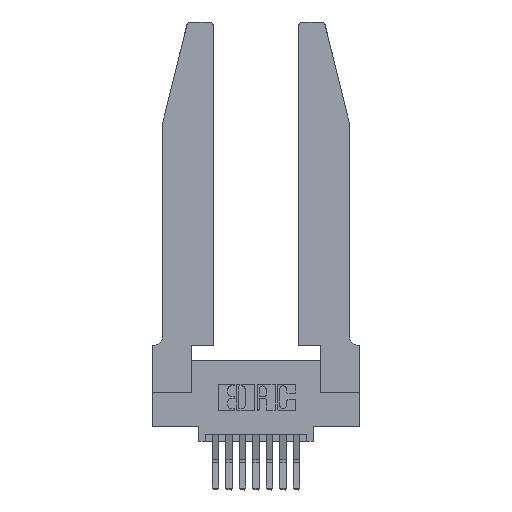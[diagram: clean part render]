
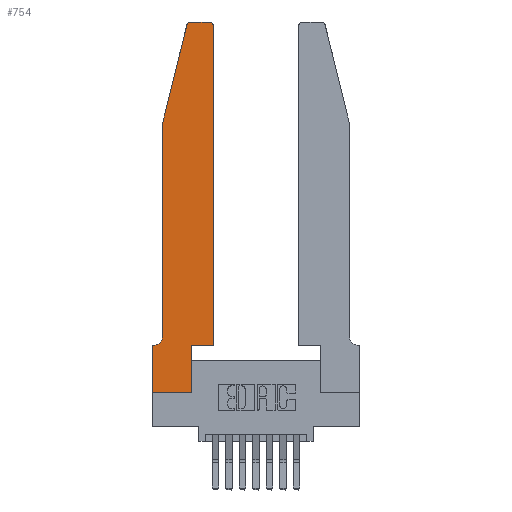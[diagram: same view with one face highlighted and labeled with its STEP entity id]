
A CAD part, top view. The second image highlights one B-rep face of the part: STEP entity #754.
In plain terms, the highlighted planar face has unit normal (0, 0, 1).
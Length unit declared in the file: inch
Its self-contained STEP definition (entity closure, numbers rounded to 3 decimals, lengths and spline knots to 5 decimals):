
#336 = VERTEX_POINT ( 'NONE', #6497 ) ;
#641 = ORIENTED_EDGE ( 'NONE', *, *, #11250, .T. ) ;
#754 = ADVANCED_FACE ( 'NONE', ( #6188 ), #2281, .T. ) ;
#1033 = ORIENTED_EDGE ( 'NONE', *, *, #3215, .T. ) ;
#1109 = EDGE_CURVE ( 'NONE', #2822, #13515, #5227, .T. ) ;
#1657 = CARTESIAN_POINT ( 'NONE',  ( 0.25487, 2.72718, 0.37 ) ) ;
#1688 = CARTESIAN_POINT ( 'NONE',  ( 0.0755, 0.35, 0.37 ) ) ;
#1771 = CARTESIAN_POINT ( 'NONE',  ( 0.4505, 0.35, 0.37 ) ) ;
#2052 = CARTESIAN_POINT ( 'NONE',  ( 0.4505, 2.72, 0.37 ) ) ;
#2219 = DIRECTION ( 'NONE',  ( 0., 0., -1. ) ) ;
#2222 = DIRECTION ( 'NONE',  ( 0., 0., 1. ) ) ;
#2240 = VECTOR ( 'NONE', #10728, 39.37008 ) ;
#2281 = PLANE ( 'NONE',  #11342 ) ;
#2646 = CARTESIAN_POINT ( 'NONE',  ( 0.284, 2.72, 0.37 ) ) ;
#2689 = VERTEX_POINT ( 'NONE', #2052 ) ;
#2822 = VERTEX_POINT ( 'NONE', #8727 ) ;
#2857 = CARTESIAN_POINT ( 'NONE',  ( 0., 0., 0.37 ) ) ;
#2932 = CARTESIAN_POINT ( 'NONE',  ( 0.4505, 0.35, 0.37 ) ) ;
#3115 = VERTEX_POINT ( 'NONE', #13414 ) ;
#3215 = EDGE_CURVE ( 'NONE', #3642, #12084, #13689, .T. ) ;
#3252 = CARTESIAN_POINT ( 'NONE',  ( 0.4205, 2.72, 0.37 ) ) ;
#3642 = VERTEX_POINT ( 'NONE', #1657 ) ;
#3873 = DIRECTION ( 'NONE',  ( 1., 0., 0. ) ) ;
#3960 = CARTESIAN_POINT ( 'NONE',  ( 0.4505, 0.35, 0.37 ) ) ;
#3964 = DIRECTION ( 'NONE',  ( 0., -1., 0. ) ) ;
#4013 = DIRECTION ( 'NONE',  ( 1., 0., 0. ) ) ;
#4084 = CIRCLE ( 'NONE', #13754, 0.03 ) ;
#4226 = ORIENTED_EDGE ( 'NONE', *, *, #5120, .T. ) ;
#4238 = CARTESIAN_POINT ( 'NONE',  ( 0.0055, 0.35, 0.37 ) ) ;
#4379 = LINE ( 'NONE', #8382, #13118 ) ;
#4435 = CARTESIAN_POINT ( 'NONE',  ( 0.2605, 2.75, 0.37 ) ) ;
#4442 = EDGE_CURVE ( 'NONE', #12084, #2822, #4379, .T. ) ;
#4458 = DIRECTION ( 'NONE',  ( 1., 0., 0. ) ) ;
#4613 = VECTOR ( 'NONE', #11310, 39.37008 ) ;
#4625 = VERTEX_POINT ( 'NONE', #10984 ) ;
#5120 = EDGE_CURVE ( 'NONE', #4625, #336, #8622, .T. ) ;
#5227 = CIRCLE ( 'NONE', #13986, 0.07 ) ;
#5838 = EDGE_CURVE ( 'NONE', #336, #7082, #13028, .T. ) ;
#5891 = VERTEX_POINT ( 'NONE', #2857 ) ;
#6188 = FACE_OUTER_BOUND ( 'NONE', #10851, .T. ) ;
#6319 = ORIENTED_EDGE ( 'NONE', *, *, #14062, .T. ) ;
#6497 = CARTESIAN_POINT ( 'NONE',  ( 0.2865, 0.35, 0.37 ) ) ;
#6561 = EDGE_CURVE ( 'NONE', #7082, #2689, #7243, .T. ) ;
#6595 = LINE ( 'NONE', #10935, #12585 ) ;
#6821 = DIRECTION ( 'NONE',  ( -1., 0., 0. ) ) ;
#6855 = CARTESIAN_POINT ( 'NONE',  ( 0.0755, 2., 0.37 ) ) ;
#7029 = EDGE_CURVE ( 'NONE', #7751, #3642, #7226, .T. ) ;
#7069 = CARTESIAN_POINT ( 'NONE',  ( 0.4205, 2.75, 0.37 ) ) ;
#7082 = VERTEX_POINT ( 'NONE', #2932 ) ;
#7086 = VECTOR ( 'NONE', #4013, 39.37008 ) ;
#7226 = CIRCLE ( 'NONE', #8506, 0.03 ) ;
#7243 = LINE ( 'NONE', #1771, #10285 ) ;
#7295 = CARTESIAN_POINT ( 'NONE',  ( 0.2865, 0.35, 0.37 ) ) ;
#7328 = DIRECTION ( 'NONE',  ( 1., 0., 0. ) ) ;
#7700 = LINE ( 'NONE', #1688, #13290 ) ;
#7751 = VERTEX_POINT ( 'NONE', #7919 ) ;
#7878 = CARTESIAN_POINT ( 'NONE',  ( 0.0755, 2., 0.37 ) ) ;
#7919 = CARTESIAN_POINT ( 'NONE',  ( 0.284, 2.75, 0.37 ) ) ;
#8382 = CARTESIAN_POINT ( 'NONE',  ( 0.0755, 2., 0.37 ) ) ;
#8506 = AXIS2_PLACEMENT_3D ( 'NONE', #2646, #10848, #3873 ) ;
#8622 = LINE ( 'NONE', #7295, #2240 ) ;
#8727 = CARTESIAN_POINT ( 'NONE',  ( 0.0755, 0.42, 0.37 ) ) ;
#8882 = VERTEX_POINT ( 'NONE', #7069 ) ;
#9174 = LINE ( 'NONE', #11056, #14657 ) ;
#9280 = EDGE_CURVE ( 'NONE', #5891, #4625, #9174, .T. ) ;
#9311 = VECTOR ( 'NONE', #11351, 39.37008 ) ;
#9752 = ORIENTED_EDGE ( 'NONE', *, *, #13910, .T. ) ;
#9962 = DIRECTION ( 'NONE',  ( 1., 0., 0. ) ) ;
#10094 = ORIENTED_EDGE ( 'NONE', *, *, #9280, .T. ) ;
#10150 = DIRECTION ( 'NONE',  ( 0., 1., 0. ) ) ;
#10285 = VECTOR ( 'NONE', #10150, 39.37008 ) ;
#10647 = DIRECTION ( 'NONE',  ( 0., -1., 0. ) ) ;
#10728 = DIRECTION ( 'NONE',  ( 0., 1., 0. ) ) ;
#10848 = DIRECTION ( 'NONE',  ( 0., 0., 1. ) ) ;
#10851 = EDGE_LOOP ( 'NONE', ( #641, #13159, #1033, #14184, #14514, #6319, #9752, #10094, #4226, #13699, #11124, #14018 ) ) ;
#10935 = CARTESIAN_POINT ( 'NONE',  ( 0., 0., 0.37 ) ) ;
#10984 = CARTESIAN_POINT ( 'NONE',  ( 0.2865, 0., 0.37 ) ) ;
#11056 = CARTESIAN_POINT ( 'NONE',  ( 0., 0., 0.37 ) ) ;
#11124 = ORIENTED_EDGE ( 'NONE', *, *, #6561, .T. ) ;
#11250 = EDGE_CURVE ( 'NONE', #8882, #7751, #12207, .T. ) ;
#11310 = DIRECTION ( 'NONE',  ( -0.239, -0.971, 0. ) ) ;
#11342 = AXIS2_PLACEMENT_3D ( 'NONE', #15188, #2222, #7328 ) ;
#11351 = DIRECTION ( 'NONE',  ( -1., 0., 0. ) ) ;
#11370 = DIRECTION ( 'NONE',  ( 0., 0., 1. ) ) ;
#12084 = VERTEX_POINT ( 'NONE', #7878 ) ;
#12123 = EDGE_CURVE ( 'NONE', #2689, #8882, #4084, .T. ) ;
#12207 = LINE ( 'NONE', #4435, #9311 ) ;
#12585 = VECTOR ( 'NONE', #3964, 39.37008 ) ;
#13028 = LINE ( 'NONE', #3960, #7086 ) ;
#13118 = VECTOR ( 'NONE', #10647, 39.37008 ) ;
#13159 = ORIENTED_EDGE ( 'NONE', *, *, #7029, .T. ) ;
#13290 = VECTOR ( 'NONE', #13377, 39.37008 ) ;
#13377 = DIRECTION ( 'NONE',  ( -1., 0., 0. ) ) ;
#13414 = CARTESIAN_POINT ( 'NONE',  ( 0., 0.35, 0.37 ) ) ;
#13515 = VERTEX_POINT ( 'NONE', #4238 ) ;
#13689 = LINE ( 'NONE', #6855, #4613 ) ;
#13699 = ORIENTED_EDGE ( 'NONE', *, *, #5838, .T. ) ;
#13754 = AXIS2_PLACEMENT_3D ( 'NONE', #3252, #11370, #4458 ) ;
#13910 = EDGE_CURVE ( 'NONE', #3115, #5891, #6595, .T. ) ;
#13986 = AXIS2_PLACEMENT_3D ( 'NONE', #15058, #2219, #6821 ) ;
#14018 = ORIENTED_EDGE ( 'NONE', *, *, #12123, .T. ) ;
#14062 = EDGE_CURVE ( 'NONE', #13515, #3115, #7700, .T. ) ;
#14184 = ORIENTED_EDGE ( 'NONE', *, *, #4442, .T. ) ;
#14514 = ORIENTED_EDGE ( 'NONE', *, *, #1109, .T. ) ;
#14657 = VECTOR ( 'NONE', #9962, 39.37008 ) ;
#15058 = CARTESIAN_POINT ( 'NONE',  ( 0.0055, 0.42, 0.37 ) ) ;
#15188 = CARTESIAN_POINT ( 'NONE',  ( 0., 0.35, 0.37 ) ) ;
